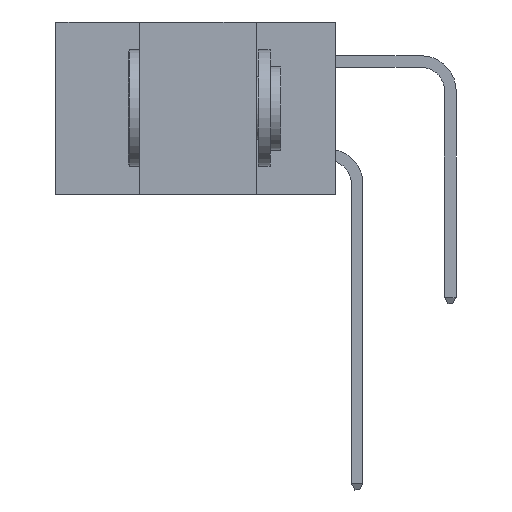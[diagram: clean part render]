
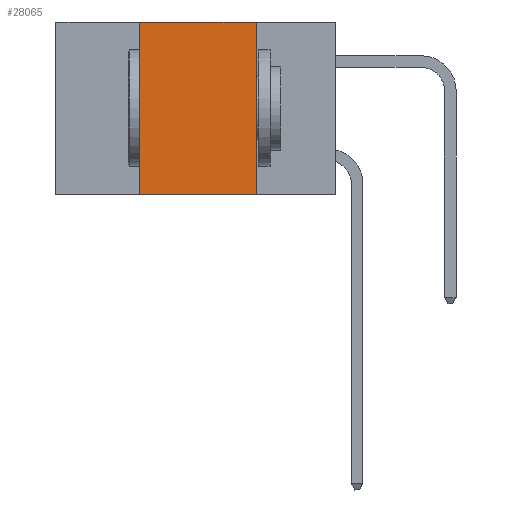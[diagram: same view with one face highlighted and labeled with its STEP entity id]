
A CAD part, left-side view. The second image highlights one B-rep face of the part: STEP entity #28065.
In plain terms, the highlighted planar face has unit normal (-1, 0, 0).
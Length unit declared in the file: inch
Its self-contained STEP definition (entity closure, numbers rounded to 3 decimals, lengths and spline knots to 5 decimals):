
#96 = CARTESIAN_POINT ( 'NONE',  ( 0., 0.17, -0.37 ) ) ;
#2809 = VERTEX_POINT ( 'NONE', #96 ) ;
#3440 = VECTOR ( 'NONE', #38315, 39.37008 ) ;
#4138 = CARTESIAN_POINT ( 'NONE',  ( 0., 0.17, 0. ) ) ;
#4773 = CARTESIAN_POINT ( 'NONE',  ( 0., 0.42, 0. ) ) ;
#4906 = VECTOR ( 'NONE', #6149, 39.37008 ) ;
#6149 = DIRECTION ( 'NONE',  ( 0., 0., -1. ) ) ;
#7919 = ORIENTED_EDGE ( 'NONE', *, *, #16366, .T. ) ;
#8947 = DIRECTION ( 'NONE',  ( 0., -1., 0. ) ) ;
#9400 = CARTESIAN_POINT ( 'NONE',  ( 0., 0.17, 0. ) ) ;
#9903 = EDGE_CURVE ( 'NONE', #21748, #31679, #33499, .T. ) ;
#12511 = CARTESIAN_POINT ( 'NONE',  ( 0., 0.6, 0. ) ) ;
#12666 = EDGE_CURVE ( 'NONE', #31679, #24254, #38981, .T. ) ;
#13673 = VECTOR ( 'NONE', #8947, 39.37008 ) ;
#13819 = LINE ( 'NONE', #9400, #4906 ) ;
#16007 = DIRECTION ( 'NONE',  ( 0., 0., -1. ) ) ;
#16366 = EDGE_CURVE ( 'NONE', #21748, #2809, #30409, .T. ) ;
#21230 = EDGE_CURVE ( 'NONE', #24254, #2809, #13819, .T. ) ;
#21748 = VERTEX_POINT ( 'NONE', #32899 ) ;
#22534 = ORIENTED_EDGE ( 'NONE', *, *, #12666, .F. ) ;
#24254 = VERTEX_POINT ( 'NONE', #4138 ) ;
#28065 = ADVANCED_FACE ( 'NONE', ( #40195 ), #32677, .F. ) ;
#28323 = ORIENTED_EDGE ( 'NONE', *, *, #21230, .F. ) ;
#28963 = CARTESIAN_POINT ( 'NONE',  ( 0., 0.6, -0.37 ) ) ;
#30034 = DIRECTION ( 'NONE',  ( 0., 0., 1. ) ) ;
#30139 = EDGE_LOOP ( 'NONE', ( #28323, #22534, #31475, #7919 ) ) ;
#30409 = LINE ( 'NONE', #28963, #13673 ) ;
#31475 = ORIENTED_EDGE ( 'NONE', *, *, #9903, .F. ) ;
#31679 = VERTEX_POINT ( 'NONE', #4773 ) ;
#32677 = PLANE ( 'NONE',  #42417 ) ;
#32899 = CARTESIAN_POINT ( 'NONE',  ( 0., 0.42, -0.37 ) ) ;
#33499 = LINE ( 'NONE', #36568, #39141 ) ;
#35039 = CARTESIAN_POINT ( 'NONE',  ( 0., 0.6, 0. ) ) ;
#36001 = DIRECTION ( 'NONE',  ( 1., 0., 0. ) ) ;
#36568 = CARTESIAN_POINT ( 'NONE',  ( 0., 0.42, 0. ) ) ;
#38315 = DIRECTION ( 'NONE',  ( 0., -1., 0. ) ) ;
#38981 = LINE ( 'NONE', #35039, #3440 ) ;
#39141 = VECTOR ( 'NONE', #30034, 39.37008 ) ;
#40195 = FACE_OUTER_BOUND ( 'NONE', #30139, .T. ) ;
#42417 = AXIS2_PLACEMENT_3D ( 'NONE', #12511, #36001, #16007 ) ;
